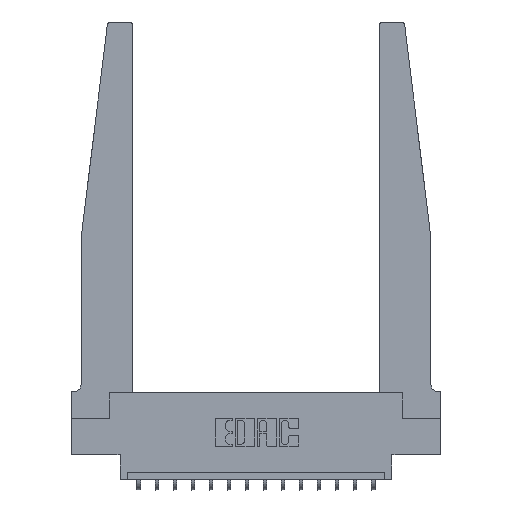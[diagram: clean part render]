
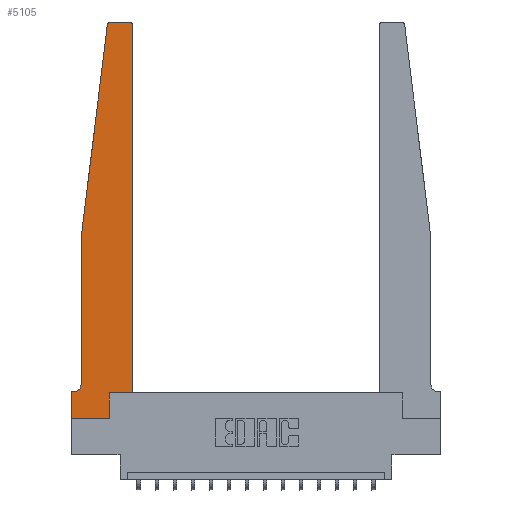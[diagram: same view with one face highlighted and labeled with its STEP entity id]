
A CAD part, top view. The second image highlights one B-rep face of the part: STEP entity #5105.
In plain terms, the highlighted planar face has unit normal (0, 0, 1).
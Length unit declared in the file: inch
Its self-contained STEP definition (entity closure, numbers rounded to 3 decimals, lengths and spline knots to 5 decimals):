
#112 = CARTESIAN_POINT ( 'NONE',  ( 0., 0., 0.37 ) ) ;
#268 = CIRCLE ( 'NONE', #17294, 0.05 ) ;
#338 = VECTOR ( 'NONE', #2301, 39.37008 ) ;
#387 = ORIENTED_EDGE ( 'NONE', *, *, #3799, .T. ) ;
#553 = VERTEX_POINT ( 'NONE', #11180 ) ;
#687 = VECTOR ( 'NONE', #17343, 39.37008 ) ;
#1077 = LINE ( 'NONE', #10748, #687 ) ;
#1102 = VECTOR ( 'NONE', #2829, 39.37008 ) ;
#1277 = EDGE_CURVE ( 'NONE', #10197, #6410, #268, .T. ) ;
#1323 = EDGE_LOOP ( 'NONE', ( #14417, #9605, #7964, #4805, #3009, #387, #14505, #10247, #9285, #8927, #17277, #4257 ) ) ;
#1731 = EDGE_CURVE ( 'NONE', #14536, #2342, #15438, .T. ) ;
#2195 = CARTESIAN_POINT ( 'NONE',  ( 0.2605, 0.18, 0.37 ) ) ;
#2301 = DIRECTION ( 'NONE',  ( -0.122, -0.992, 0. ) ) ;
#2342 = VERTEX_POINT ( 'NONE', #15677 ) ;
#2355 = DIRECTION ( 'NONE',  ( -1., 0., 0. ) ) ;
#2670 = CARTESIAN_POINT ( 'NONE',  ( 0.065, 1.25, 0.37 ) ) ;
#2764 = LINE ( 'NONE', #16674, #3435 ) ;
#2829 = DIRECTION ( 'NONE',  ( 1., 0., 0. ) ) ;
#2866 = DIRECTION ( 'NONE',  ( 1., 0., 0. ) ) ;
#2954 = LINE ( 'NONE', #2670, #3994 ) ;
#3009 = ORIENTED_EDGE ( 'NONE', *, *, #1277, .T. ) ;
#3105 = CIRCLE ( 'NONE', #5699, 0.03 ) ;
#3138 = CARTESIAN_POINT ( 'NONE',  ( 0.065, 0.2375, 0.37 ) ) ;
#3435 = VECTOR ( 'NONE', #3934, 39.37008 ) ;
#3660 = LINE ( 'NONE', #9185, #338 ) ;
#3799 = EDGE_CURVE ( 'NONE', #6410, #16337, #14975, .T. ) ;
#3934 = DIRECTION ( 'NONE',  ( 0., 1., 0. ) ) ;
#3994 = VECTOR ( 'NONE', #14959, 39.37008 ) ;
#4217 = EDGE_CURVE ( 'NONE', #5180, #11680, #3660, .T. ) ;
#4257 = ORIENTED_EDGE ( 'NONE', *, *, #12280, .T. ) ;
#4341 = CARTESIAN_POINT ( 'NONE',  ( 0.015, 0.1875, 0.37 ) ) ;
#4495 = EDGE_CURVE ( 'NONE', #2342, #12040, #17111, .T. ) ;
#4805 = ORIENTED_EDGE ( 'NONE', *, *, #16014, .T. ) ;
#5105 = ADVANCED_FACE ( 'NONE', ( #13453 ), #9499, .T. ) ;
#5180 = VERTEX_POINT ( 'NONE', #17529 ) ;
#5505 = DIRECTION ( 'NONE',  ( -1., 0., 0. ) ) ;
#5699 = AXIS2_PLACEMENT_3D ( 'NONE', #8953, #6149, #17241 ) ;
#5894 = CIRCLE ( 'NONE', #8199, 0.03 ) ;
#6149 = DIRECTION ( 'NONE',  ( 0., 0., 1. ) ) ;
#6410 = VERTEX_POINT ( 'NONE', #4341 ) ;
#6467 = EDGE_CURVE ( 'NONE', #12663, #5180, #5894, .T. ) ;
#6851 = CARTESIAN_POINT ( 'NONE',  ( 0.065, 0.1875, 0.37 ) ) ;
#6985 = VECTOR ( 'NONE', #12353, 39.37008 ) ;
#7168 = CARTESIAN_POINT ( 'NONE',  ( 0.065, 1.25, 0.37 ) ) ;
#7293 = CARTESIAN_POINT ( 'NONE',  ( 0.425, 0.18, 0.37 ) ) ;
#7508 = VERTEX_POINT ( 'NONE', #9107 ) ;
#7645 = CARTESIAN_POINT ( 'NONE',  ( 0.27653, 2.75, 0.37 ) ) ;
#7845 = CARTESIAN_POINT ( 'NONE',  ( 0., 0., 0.37 ) ) ;
#7964 = ORIENTED_EDGE ( 'NONE', *, *, #4217, .T. ) ;
#8061 = LINE ( 'NONE', #17721, #15549 ) ;
#8103 = DIRECTION ( 'NONE',  ( 0., 0., 1. ) ) ;
#8199 = AXIS2_PLACEMENT_3D ( 'NONE', #10032, #15554, #14102 ) ;
#8469 = EDGE_CURVE ( 'NONE', #16337, #13314, #1077, .T. ) ;
#8927 = ORIENTED_EDGE ( 'NONE', *, *, #1731, .T. ) ;
#8953 = CARTESIAN_POINT ( 'NONE',  ( 0.395, 2.72, 0.37 ) ) ;
#9107 = CARTESIAN_POINT ( 'NONE',  ( 0.2605, 0., 0.37 ) ) ;
#9185 = CARTESIAN_POINT ( 'NONE',  ( 0.065, 1.25, 0.37 ) ) ;
#9285 = ORIENTED_EDGE ( 'NONE', *, *, #16064, .T. ) ;
#9499 = PLANE ( 'NONE',  #16535 ) ;
#9605 = ORIENTED_EDGE ( 'NONE', *, *, #6467, .T. ) ;
#9616 = LINE ( 'NONE', #112, #1102 ) ;
#10032 = CARTESIAN_POINT ( 'NONE',  ( 0.27653, 2.72, 0.37 ) ) ;
#10197 = VERTEX_POINT ( 'NONE', #3138 ) ;
#10247 = ORIENTED_EDGE ( 'NONE', *, *, #14740, .T. ) ;
#10413 = VECTOR ( 'NONE', #2866, 39.37008 ) ;
#10748 = CARTESIAN_POINT ( 'NONE',  ( 0., 0., 0.37 ) ) ;
#10847 = DIRECTION ( 'NONE',  ( 0., 0., -1. ) ) ;
#10937 = CARTESIAN_POINT ( 'NONE',  ( 0.015, 0.2375, 0.37 ) ) ;
#11180 = CARTESIAN_POINT ( 'NONE',  ( 0.395, 2.75, 0.37 ) ) ;
#11439 = DIRECTION ( 'NONE',  ( 0., 1., 0. ) ) ;
#11680 = VERTEX_POINT ( 'NONE', #7168 ) ;
#12040 = VERTEX_POINT ( 'NONE', #16367 ) ;
#12280 = EDGE_CURVE ( 'NONE', #12040, #553, #3105, .T. ) ;
#12353 = DIRECTION ( 'NONE',  ( -1., 0., 0. ) ) ;
#12652 = CARTESIAN_POINT ( 'NONE',  ( 0., 0.1875, 0.37 ) ) ;
#12663 = VERTEX_POINT ( 'NONE', #7645 ) ;
#13314 = VERTEX_POINT ( 'NONE', #7845 ) ;
#13453 = FACE_OUTER_BOUND ( 'NONE', #1323, .T. ) ;
#13541 = CARTESIAN_POINT ( 'NONE',  ( 0., 0.1875, 0.37 ) ) ;
#14102 = DIRECTION ( 'NONE',  ( 1., 0., 0. ) ) ;
#14417 = ORIENTED_EDGE ( 'NONE', *, *, #15146, .T. ) ;
#14497 = VECTOR ( 'NONE', #11439, 39.37008 ) ;
#14505 = ORIENTED_EDGE ( 'NONE', *, *, #8469, .T. ) ;
#14536 = VERTEX_POINT ( 'NONE', #2195 ) ;
#14740 = EDGE_CURVE ( 'NONE', #13314, #7508, #9616, .T. ) ;
#14959 = DIRECTION ( 'NONE',  ( 0., -1., 0. ) ) ;
#14975 = LINE ( 'NONE', #6851, #6985 ) ;
#15146 = EDGE_CURVE ( 'NONE', #553, #12663, #8061, .T. ) ;
#15438 = LINE ( 'NONE', #7293, #10413 ) ;
#15549 = VECTOR ( 'NONE', #2355, 39.37008 ) ;
#15554 = DIRECTION ( 'NONE',  ( 0., 0., 1. ) ) ;
#15677 = CARTESIAN_POINT ( 'NONE',  ( 0.425, 0.18, 0.37 ) ) ;
#16014 = EDGE_CURVE ( 'NONE', #11680, #10197, #2954, .T. ) ;
#16064 = EDGE_CURVE ( 'NONE', #7508, #14536, #2764, .T. ) ;
#16186 = DIRECTION ( 'NONE',  ( 1., 0., 0. ) ) ;
#16337 = VERTEX_POINT ( 'NONE', #12652 ) ;
#16367 = CARTESIAN_POINT ( 'NONE',  ( 0.425, 2.72, 0.37 ) ) ;
#16535 = AXIS2_PLACEMENT_3D ( 'NONE', #13541, #8103, #16186 ) ;
#16674 = CARTESIAN_POINT ( 'NONE',  ( 0.2605, 0.18, 0.37 ) ) ;
#16754 = CARTESIAN_POINT ( 'NONE',  ( 0.425, 0.18, 0.37 ) ) ;
#17111 = LINE ( 'NONE', #16754, #14497 ) ;
#17241 = DIRECTION ( 'NONE',  ( 1., 0., 0. ) ) ;
#17277 = ORIENTED_EDGE ( 'NONE', *, *, #4495, .T. ) ;
#17294 = AXIS2_PLACEMENT_3D ( 'NONE', #10937, #10847, #5505 ) ;
#17343 = DIRECTION ( 'NONE',  ( 0., -1., 0. ) ) ;
#17529 = CARTESIAN_POINT ( 'NONE',  ( 0.24675, 2.72367, 0.37 ) ) ;
#17721 = CARTESIAN_POINT ( 'NONE',  ( 0.25, 2.75, 0.37 ) ) ;
